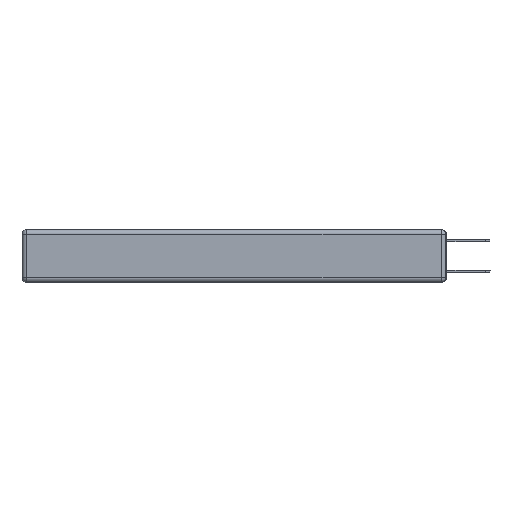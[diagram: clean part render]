
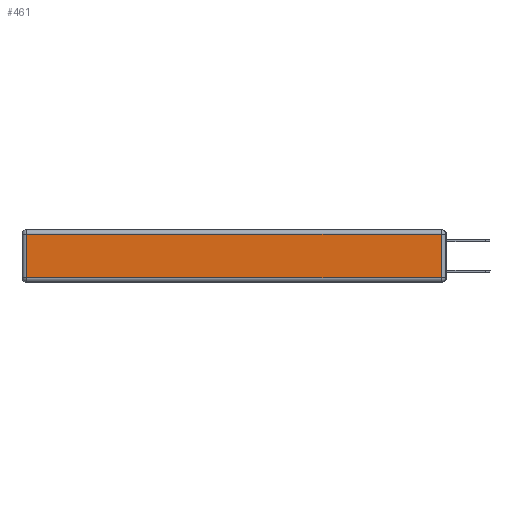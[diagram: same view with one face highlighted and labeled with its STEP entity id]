
A CAD part, left-side view. The second image highlights one B-rep face of the part: STEP entity #461.
In plain terms, the highlighted planar face has unit normal (-1, 0, 0).
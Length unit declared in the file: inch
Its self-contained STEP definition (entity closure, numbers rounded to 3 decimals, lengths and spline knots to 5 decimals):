
#44 = EDGE_CURVE ( 'NONE', #4195, #14830, #10626, .T. ) ;
#208 = ORIENTED_EDGE ( 'NONE', *, *, #6837, .T. ) ;
#220 = CARTESIAN_POINT ( 'NONE',  ( 0., 2.72, -0.313 ) ) ;
#461 = ADVANCED_FACE ( 'NONE', ( #8848 ), #10690, .T. ) ;
#2870 = VECTOR ( 'NONE', #6920, 39.37008 ) ;
#2889 = VECTOR ( 'NONE', #8002, 39.37008 ) ;
#3069 = CARTESIAN_POINT ( 'NONE',  ( 0., 0., -0.313 ) ) ;
#4049 = CARTESIAN_POINT ( 'NONE',  ( 0., 0.03, -0.313 ) ) ;
#4195 = VERTEX_POINT ( 'NONE', #13298 ) ;
#4343 = CARTESIAN_POINT ( 'NONE',  ( 0., 0., -0.343 ) ) ;
#4516 = DIRECTION ( 'NONE',  ( 0., 0., -1. ) ) ;
#6794 = LINE ( 'NONE', #3069, #2870 ) ;
#6837 = EDGE_CURVE ( 'NONE', #12418, #4195, #12761, .T. ) ;
#6890 = CARTESIAN_POINT ( 'NONE',  ( 0., 2.75, -0.03 ) ) ;
#6920 = DIRECTION ( 'NONE',  ( 0., -1., 0. ) ) ;
#7179 = CARTESIAN_POINT ( 'NONE',  ( 0., 0.03, -0.343 ) ) ;
#7691 = EDGE_CURVE ( 'NONE', #14830, #9734, #6794, .T. ) ;
#7901 = EDGE_LOOP ( 'NONE', ( #15789, #12744, #208, #9208 ) ) ;
#8002 = DIRECTION ( 'NONE',  ( 0., 1., 0. ) ) ;
#8848 = FACE_OUTER_BOUND ( 'NONE', #7901, .T. ) ;
#9208 = ORIENTED_EDGE ( 'NONE', *, *, #44, .T. ) ;
#9734 = VERTEX_POINT ( 'NONE', #4049 ) ;
#10626 = LINE ( 'NONE', #12082, #12393 ) ;
#10690 = PLANE ( 'NONE',  #13561 ) ;
#11897 = LINE ( 'NONE', #7179, #16263 ) ;
#12082 = CARTESIAN_POINT ( 'NONE',  ( 0., 2.72, -0.343 ) ) ;
#12393 = VECTOR ( 'NONE', #4516, 39.37008 ) ;
#12418 = VERTEX_POINT ( 'NONE', #12969 ) ;
#12744 = ORIENTED_EDGE ( 'NONE', *, *, #13221, .T. ) ;
#12761 = LINE ( 'NONE', #6890, #2889 ) ;
#12969 = CARTESIAN_POINT ( 'NONE',  ( 0., 0.03, -0.03 ) ) ;
#13067 = DIRECTION ( 'NONE',  ( -1., 0., 0. ) ) ;
#13129 = DIRECTION ( 'NONE',  ( 0., 0., 1. ) ) ;
#13221 = EDGE_CURVE ( 'NONE', #9734, #12418, #11897, .T. ) ;
#13298 = CARTESIAN_POINT ( 'NONE',  ( 0., 2.72, -0.03 ) ) ;
#13385 = DIRECTION ( 'NONE',  ( 0., 0., 1. ) ) ;
#13561 = AXIS2_PLACEMENT_3D ( 'NONE', #4343, #13067, #13129 ) ;
#14830 = VERTEX_POINT ( 'NONE', #220 ) ;
#15789 = ORIENTED_EDGE ( 'NONE', *, *, #7691, .T. ) ;
#16263 = VECTOR ( 'NONE', #13385, 39.37008 ) ;
